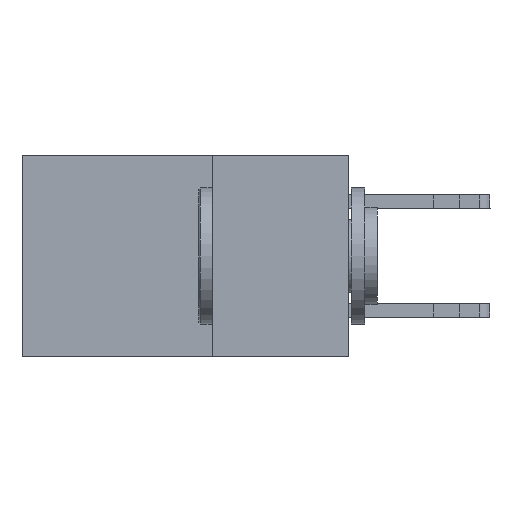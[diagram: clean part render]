
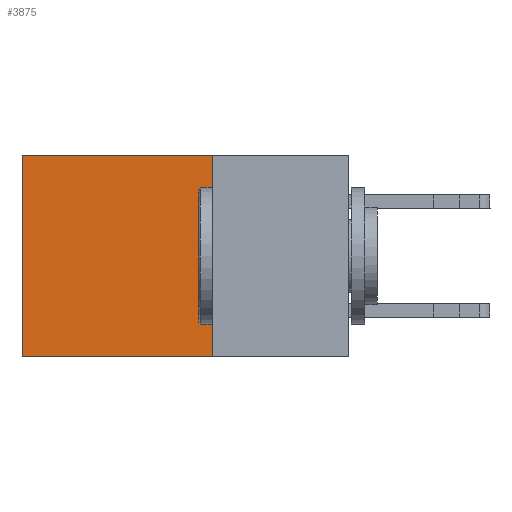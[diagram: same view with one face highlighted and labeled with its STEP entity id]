
A CAD part, left-side view. The second image highlights one B-rep face of the part: STEP entity #3875.
In plain terms, the highlighted planar face has unit normal (-1, 0, 0).
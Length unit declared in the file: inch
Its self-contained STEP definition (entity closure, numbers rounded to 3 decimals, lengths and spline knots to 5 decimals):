
#104 = CARTESIAN_POINT ( 'NONE',  ( 0.2615, 0.25, 0. ) ) ;
#553 = PLANE ( 'NONE',  #1050 ) ;
#595 = CARTESIAN_POINT ( 'NONE',  ( 0.2615, 0.25, -0.37 ) ) ;
#1050 = AXIS2_PLACEMENT_3D ( 'NONE', #4103, #8826, #12457 ) ;
#2029 = VECTOR ( 'NONE', #10904, 39.37008 ) ;
#3253 = VERTEX_POINT ( 'NONE', #10780 ) ;
#3875 = ADVANCED_FACE ( 'NONE', ( #4021 ), #553, .F. ) ;
#4021 = FACE_OUTER_BOUND ( 'NONE', #4023, .T. ) ;
#4023 = EDGE_LOOP ( 'NONE', ( #4971, #9531, #5247, #9591 ) ) ;
#4027 = LINE ( 'NONE', #12062, #2029 ) ;
#4103 = CARTESIAN_POINT ( 'NONE',  ( 0.2615, 0.25, -0.37 ) ) ;
#4571 = EDGE_CURVE ( 'NONE', #11622, #6621, #8321, .T. ) ;
#4946 = VECTOR ( 'NONE', #13109, 39.37008 ) ;
#4971 = ORIENTED_EDGE ( 'NONE', *, *, #4571, .T. ) ;
#5247 = ORIENTED_EDGE ( 'NONE', *, *, #12911, .F. ) ;
#5741 = LINE ( 'NONE', #15142, #13058 ) ;
#6128 = CARTESIAN_POINT ( 'NONE',  ( 0.2615, 0.6, -0.37 ) ) ;
#6288 = DIRECTION ( 'NONE',  ( 0., 0., -1. ) ) ;
#6304 = EDGE_CURVE ( 'NONE', #8611, #11622, #5741, .T. ) ;
#6621 = VERTEX_POINT ( 'NONE', #10314 ) ;
#6650 = CARTESIAN_POINT ( 'NONE',  ( 0.2615, 0.6, 0. ) ) ;
#8321 = LINE ( 'NONE', #6128, #4946 ) ;
#8611 = VERTEX_POINT ( 'NONE', #104 ) ;
#8826 = DIRECTION ( 'NONE',  ( 1., 0., 0. ) ) ;
#9531 = ORIENTED_EDGE ( 'NONE', *, *, #12353, .F. ) ;
#9591 = ORIENTED_EDGE ( 'NONE', *, *, #6304, .T. ) ;
#9916 = VECTOR ( 'NONE', #6288, 39.37008 ) ;
#10314 = CARTESIAN_POINT ( 'NONE',  ( 0.2615, 0.6, -0.37 ) ) ;
#10780 = CARTESIAN_POINT ( 'NONE',  ( 0.2615, 0.25, -0.37 ) ) ;
#10904 = DIRECTION ( 'NONE',  ( 0., 1., 0. ) ) ;
#11100 = LINE ( 'NONE', #595, #9916 ) ;
#11427 = DIRECTION ( 'NONE',  ( 0., 1., 0. ) ) ;
#11622 = VERTEX_POINT ( 'NONE', #6650 ) ;
#12062 = CARTESIAN_POINT ( 'NONE',  ( 0.2615, 0.25, -0.37 ) ) ;
#12353 = EDGE_CURVE ( 'NONE', #3253, #6621, #4027, .T. ) ;
#12457 = DIRECTION ( 'NONE',  ( 0., 0., -1. ) ) ;
#12911 = EDGE_CURVE ( 'NONE', #8611, #3253, #11100, .T. ) ;
#13058 = VECTOR ( 'NONE', #11427, 39.37008 ) ;
#13109 = DIRECTION ( 'NONE',  ( 0., 0., -1. ) ) ;
#15142 = CARTESIAN_POINT ( 'NONE',  ( 0.2615, 0.25, 0. ) ) ;
